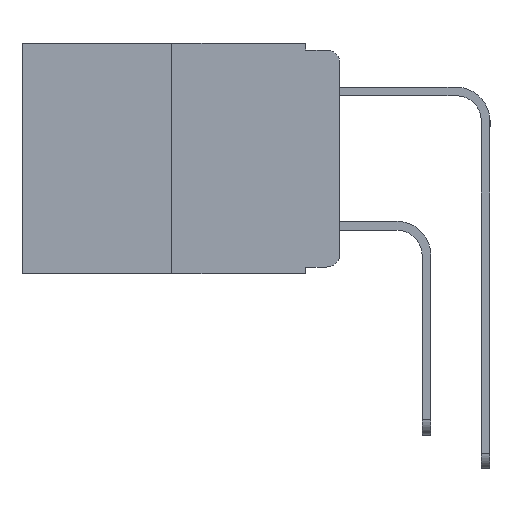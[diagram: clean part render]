
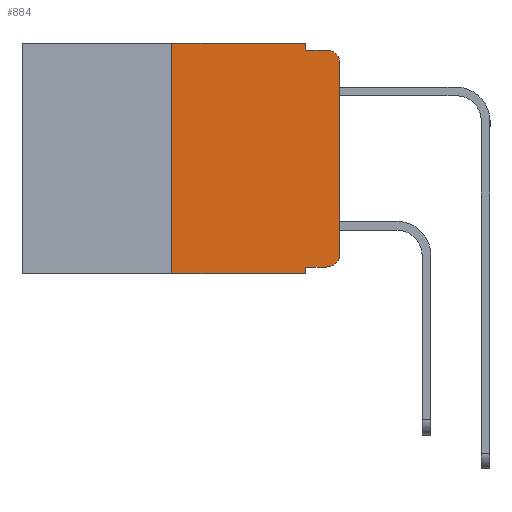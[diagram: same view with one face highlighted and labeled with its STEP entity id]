
A CAD part, left-side view. The second image highlights one B-rep face of the part: STEP entity #884.
In plain terms, the highlighted planar face has unit normal (-1, 0, 0).
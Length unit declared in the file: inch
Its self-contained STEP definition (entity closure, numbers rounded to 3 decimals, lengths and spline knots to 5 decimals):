
#477 = LINE ( 'NONE', #10031, #9408 ) ;
#506 = DIRECTION ( 'NONE',  ( -1., 0., 0. ) ) ;
#512 = EDGE_CURVE ( 'NONE', #515, #5391, #477, .T. ) ;
#515 = VERTEX_POINT ( 'NONE', #5483 ) ;
#768 = VECTOR ( 'NONE', #3057, 39.37008 ) ;
#829 = DIRECTION ( 'NONE',  ( 1., 0., 0. ) ) ;
#884 = ADVANCED_FACE ( 'NONE', ( #11722 ), #13034, .F. ) ;
#901 = DIRECTION ( 'NONE',  ( 0., 0., 1. ) ) ;
#1030 = CARTESIAN_POINT ( 'NONE',  ( 0., 0.473, -0.343 ) ) ;
#1081 = CARTESIAN_POINT ( 'NONE',  ( 0., 0.051, -0.343 ) ) ;
#1084 = CARTESIAN_POINT ( 'NONE',  ( 0., 0.473, 0. ) ) ;
#1307 = ORIENTED_EDGE ( 'NONE', *, *, #13477, .F. ) ;
#1638 = CARTESIAN_POINT ( 'NONE',  ( 0., 0.051, 0. ) ) ;
#2187 = CARTESIAN_POINT ( 'NONE',  ( 0., 0.051, -0.01 ) ) ;
#2305 = EDGE_CURVE ( 'NONE', #13700, #12882, #9567, .T. ) ;
#2549 = CARTESIAN_POINT ( 'NONE',  ( 0., 0.25, 0. ) ) ;
#2618 = LINE ( 'NONE', #9097, #11094 ) ;
#2638 = DIRECTION ( 'NONE',  ( 0., 0., -1. ) ) ;
#2762 = DIRECTION ( 'NONE',  ( 0., 0., -1. ) ) ;
#2865 = CARTESIAN_POINT ( 'NONE',  ( 0., 0.02, -0.313 ) ) ;
#3057 = DIRECTION ( 'NONE',  ( 0., -1., 0. ) ) ;
#3534 = VECTOR ( 'NONE', #6180, 39.37008 ) ;
#3665 = AXIS2_PLACEMENT_3D ( 'NONE', #7742, #506, #8774 ) ;
#3727 = CARTESIAN_POINT ( 'NONE',  ( 0., 0.25, -0.343 ) ) ;
#3778 = ORIENTED_EDGE ( 'NONE', *, *, #7049, .T. ) ;
#3840 = EDGE_CURVE ( 'NONE', #8315, #5945, #11041, .T. ) ;
#3869 = VERTEX_POINT ( 'NONE', #1638 ) ;
#4066 = DIRECTION ( 'NONE',  ( 0., -1., 0. ) ) ;
#4084 = DIRECTION ( 'NONE',  ( 0., 0., -1. ) ) ;
#4158 = ORIENTED_EDGE ( 'NONE', *, *, #3840, .F. ) ;
#4185 = VERTEX_POINT ( 'NONE', #13145 ) ;
#4346 = EDGE_CURVE ( 'NONE', #515, #12882, #9818, .T. ) ;
#4520 = EDGE_LOOP ( 'NONE', ( #3778, #12405, #4158, #10067, #12737, #1307, #7714, #10355, #8041, #13378 ) ) ;
#4735 = LINE ( 'NONE', #7063, #13216 ) ;
#4743 = VERTEX_POINT ( 'NONE', #2549 ) ;
#5391 = VERTEX_POINT ( 'NONE', #10481 ) ;
#5483 = CARTESIAN_POINT ( 'NONE',  ( 0., 0.051, -0.333 ) ) ;
#5626 = EDGE_CURVE ( 'NONE', #4743, #3869, #9641, .T. ) ;
#5945 = VERTEX_POINT ( 'NONE', #9573 ) ;
#6180 = DIRECTION ( 'NONE',  ( 0., -1., 0. ) ) ;
#6763 = EDGE_CURVE ( 'NONE', #7323, #5945, #10970, .T. ) ;
#7049 = EDGE_CURVE ( 'NONE', #4185, #7323, #4735, .T. ) ;
#7063 = CARTESIAN_POINT ( 'NONE',  ( 0., 0., 0. ) ) ;
#7323 = VERTEX_POINT ( 'NONE', #11518 ) ;
#7702 = AXIS2_PLACEMENT_3D ( 'NONE', #2865, #10638, #4084 ) ;
#7714 = ORIENTED_EDGE ( 'NONE', *, *, #2305, .T. ) ;
#7742 = CARTESIAN_POINT ( 'NONE',  ( 0., 0.02, -0.03 ) ) ;
#8041 = ORIENTED_EDGE ( 'NONE', *, *, #512, .T. ) ;
#8315 = VERTEX_POINT ( 'NONE', #2187 ) ;
#8488 = LINE ( 'NONE', #10452, #13851 ) ;
#8774 = DIRECTION ( 'NONE',  ( 0., 0., -1. ) ) ;
#9097 = CARTESIAN_POINT ( 'NONE',  ( 0., 0.25, 0. ) ) ;
#9408 = VECTOR ( 'NONE', #13688, 39.37008 ) ;
#9567 = LINE ( 'NONE', #1030, #3534 ) ;
#9573 = CARTESIAN_POINT ( 'NONE',  ( 0., 0.02, -0.01 ) ) ;
#9641 = LINE ( 'NONE', #9825, #768 ) ;
#9792 = EDGE_CURVE ( 'NONE', #5391, #4185, #12620, .T. ) ;
#9818 = LINE ( 'NONE', #13912, #12157 ) ;
#9825 = CARTESIAN_POINT ( 'NONE',  ( 0., 0.473, 0. ) ) ;
#10031 = CARTESIAN_POINT ( 'NONE',  ( 0., 0.051, -0.333 ) ) ;
#10067 = ORIENTED_EDGE ( 'NONE', *, *, #13060, .F. ) ;
#10355 = ORIENTED_EDGE ( 'NONE', *, *, #4346, .F. ) ;
#10452 = CARTESIAN_POINT ( 'NONE',  ( 0., 0.051, 0. ) ) ;
#10481 = CARTESIAN_POINT ( 'NONE',  ( 0., 0.02, -0.333 ) ) ;
#10638 = DIRECTION ( 'NONE',  ( -1., 0., 0. ) ) ;
#10970 = CIRCLE ( 'NONE', #3665, 0.02 ) ;
#11041 = LINE ( 'NONE', #11580, #11364 ) ;
#11094 = VECTOR ( 'NONE', #901, 39.37008 ) ;
#11364 = VECTOR ( 'NONE', #4066, 39.37008 ) ;
#11518 = CARTESIAN_POINT ( 'NONE',  ( 0., 0., -0.03 ) ) ;
#11580 = CARTESIAN_POINT ( 'NONE',  ( 0., 0.051, -0.01 ) ) ;
#11722 = FACE_OUTER_BOUND ( 'NONE', #4520, .T. ) ;
#12157 = VECTOR ( 'NONE', #12927, 39.37008 ) ;
#12405 = ORIENTED_EDGE ( 'NONE', *, *, #6763, .T. ) ;
#12620 = CIRCLE ( 'NONE', #7702, 0.02 ) ;
#12737 = ORIENTED_EDGE ( 'NONE', *, *, #5626, .F. ) ;
#12766 = AXIS2_PLACEMENT_3D ( 'NONE', #1084, #829, #2762 ) ;
#12882 = VERTEX_POINT ( 'NONE', #1081 ) ;
#12927 = DIRECTION ( 'NONE',  ( 0., 0., -1. ) ) ;
#13034 = PLANE ( 'NONE',  #12766 ) ;
#13060 = EDGE_CURVE ( 'NONE', #3869, #8315, #8488, .T. ) ;
#13145 = CARTESIAN_POINT ( 'NONE',  ( 0., 0., -0.313 ) ) ;
#13216 = VECTOR ( 'NONE', #14221, 39.37008 ) ;
#13378 = ORIENTED_EDGE ( 'NONE', *, *, #9792, .T. ) ;
#13477 = EDGE_CURVE ( 'NONE', #13700, #4743, #2618, .T. ) ;
#13688 = DIRECTION ( 'NONE',  ( 0., -1., 0. ) ) ;
#13700 = VERTEX_POINT ( 'NONE', #3727 ) ;
#13851 = VECTOR ( 'NONE', #2638, 39.37008 ) ;
#13912 = CARTESIAN_POINT ( 'NONE',  ( 0., 0.051, 0. ) ) ;
#14221 = DIRECTION ( 'NONE',  ( 0., 0., 1. ) ) ;
